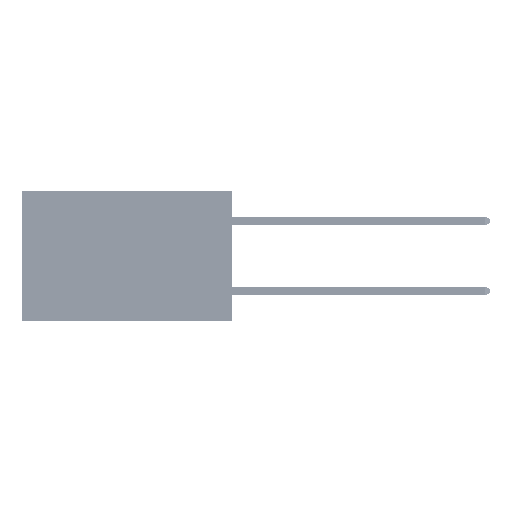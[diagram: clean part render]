
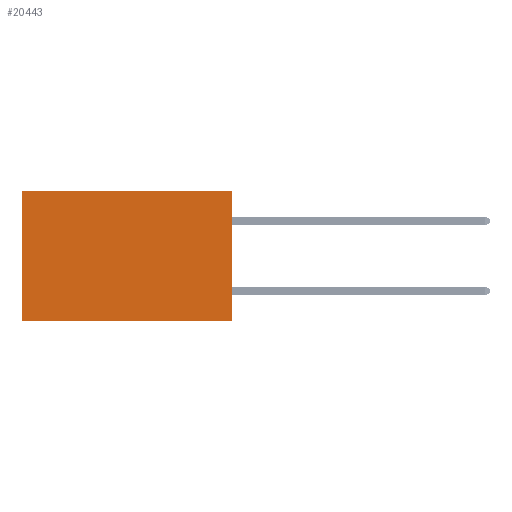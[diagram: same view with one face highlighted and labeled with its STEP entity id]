
A CAD part, left-side view. The second image highlights one B-rep face of the part: STEP entity #20443.
In plain terms, the highlighted planar face has unit normal (-1, 0, 0).
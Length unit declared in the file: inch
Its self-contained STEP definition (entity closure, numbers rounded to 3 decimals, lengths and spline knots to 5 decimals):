
#59 = CARTESIAN_POINT ( 'NONE',  ( 0.2875, 0., -0.37 ) ) ;
#594 = LINE ( 'NONE', #43394, #13629 ) ;
#2285 = EDGE_CURVE ( 'NONE', #42600, #9499, #35561, .T. ) ;
#2701 = FACE_OUTER_BOUND ( 'NONE', #8330, .T. ) ;
#2973 = EDGE_CURVE ( 'NONE', #42600, #44089, #594, .T. ) ;
#8330 = EDGE_LOOP ( 'NONE', ( #13146, #37615, #12825, #33539 ) ) ;
#8430 = DIRECTION ( 'NONE',  ( 1., 0., 0. ) ) ;
#8766 = DIRECTION ( 'NONE',  ( 0., 0., -1. ) ) ;
#9499 = VERTEX_POINT ( 'NONE', #29519 ) ;
#10329 = LINE ( 'NONE', #59, #32778 ) ;
#12564 = PLANE ( 'NONE',  #26540 ) ;
#12825 = ORIENTED_EDGE ( 'NONE', *, *, #2285, .F. ) ;
#13146 = ORIENTED_EDGE ( 'NONE', *, *, #43766, .T. ) ;
#13629 = VECTOR ( 'NONE', #24909, 39.37008 ) ;
#16062 = CARTESIAN_POINT ( 'NONE',  ( 0.2875, 0., 0. ) ) ;
#19038 = DIRECTION ( 'NONE',  ( 0., 0., -1. ) ) ;
#20443 = ADVANCED_FACE ( 'NONE', ( #2701 ), #12564, .F. ) ;
#24909 = DIRECTION ( 'NONE',  ( 0., 1., 0. ) ) ;
#26540 = AXIS2_PLACEMENT_3D ( 'NONE', #16062, #8430, #8766 ) ;
#29519 = CARTESIAN_POINT ( 'NONE',  ( 0.2875, 0., -0.37 ) ) ;
#29975 = DIRECTION ( 'NONE',  ( 0., 0., -1. ) ) ;
#30938 = EDGE_CURVE ( 'NONE', #9499, #44834, #10329, .T. ) ;
#32778 = VECTOR ( 'NONE', #33791, 39.37008 ) ;
#33539 = ORIENTED_EDGE ( 'NONE', *, *, #2973, .T. ) ;
#33791 = DIRECTION ( 'NONE',  ( 0., 1., 0. ) ) ;
#34429 = CARTESIAN_POINT ( 'NONE',  ( 0.2875, 0., 0. ) ) ;
#35561 = LINE ( 'NONE', #34429, #44438 ) ;
#37615 = ORIENTED_EDGE ( 'NONE', *, *, #30938, .F. ) ;
#37622 = VECTOR ( 'NONE', #29975, 39.37008 ) ;
#40340 = CARTESIAN_POINT ( 'NONE',  ( 0.2875, 0.6, -0.37 ) ) ;
#42401 = LINE ( 'NONE', #48649, #37622 ) ;
#42600 = VERTEX_POINT ( 'NONE', #45352 ) ;
#43394 = CARTESIAN_POINT ( 'NONE',  ( 0.2875, 0., 0. ) ) ;
#43766 = EDGE_CURVE ( 'NONE', #44089, #44834, #42401, .T. ) ;
#44089 = VERTEX_POINT ( 'NONE', #46315 ) ;
#44438 = VECTOR ( 'NONE', #19038, 39.37008 ) ;
#44834 = VERTEX_POINT ( 'NONE', #40340 ) ;
#45352 = CARTESIAN_POINT ( 'NONE',  ( 0.2875, 0., 0. ) ) ;
#46315 = CARTESIAN_POINT ( 'NONE',  ( 0.2875, 0.6, 0. ) ) ;
#48649 = CARTESIAN_POINT ( 'NONE',  ( 0.2875, 0.6, 0. ) ) ;
